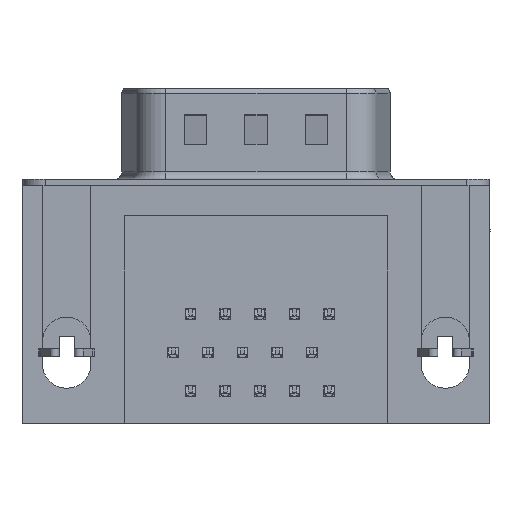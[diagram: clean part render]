
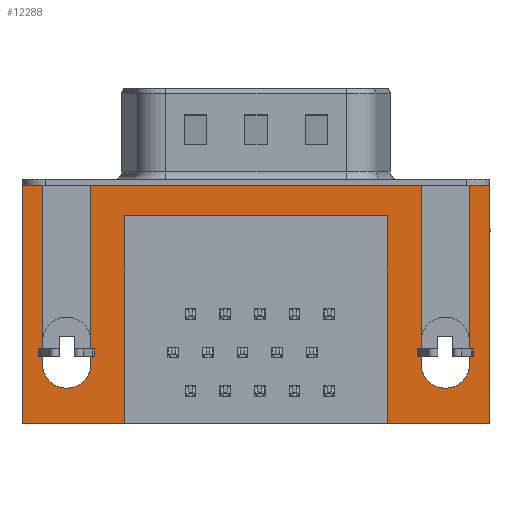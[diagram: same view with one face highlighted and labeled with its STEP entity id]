
A CAD part, front view. The second image highlights one B-rep face of the part: STEP entity #12288.
In plain terms, the highlighted planar face has unit normal (0, -1, 0).
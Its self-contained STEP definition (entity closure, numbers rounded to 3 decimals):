
#37 = DIRECTION ( 'NONE',  ( -1., 0., 0. ) ) ;
#193 = DIRECTION ( 'NONE',  ( 0., 0., 1. ) ) ;
#210 = CARTESIAN_POINT ( 'NONE',  ( 27.9, -6.275, -15.7 ) ) ;
#268 = DIRECTION ( 'NONE',  ( 1., 0., 0. ) ) ;
#341 = CARTESIAN_POINT ( 'NONE',  ( 1.6, -6.275, 0. ) ) ;
#357 = CARTESIAN_POINT ( 'NONE',  ( -2.91, -6.275, -2.5 ) ) ;
#441 = ORIENTED_EDGE ( 'NONE', *, *, #8083, .F. ) ;
#498 = LINE ( 'NONE', #14745, #18078 ) ;
#510 = DIRECTION ( 'NONE',  ( 0., -1., 0. ) ) ;
#714 = VECTOR ( 'NONE', #10806, 1000. ) ;
#1079 = VECTOR ( 'NONE', #17874, 1000. ) ;
#1080 = ORIENTED_EDGE ( 'NONE', *, *, #13354, .F. ) ;
#1344 = CARTESIAN_POINT ( 'NONE',  ( 27.9, -6.275, 0. ) ) ;
#1363 = DIRECTION ( 'NONE',  ( 0., 0., 1. ) ) ;
#1400 = EDGE_CURVE ( 'NONE', #19019, #16526, #22117, .T. ) ;
#1533 = ORIENTED_EDGE ( 'NONE', *, *, #7361, .F. ) ;
#1946 = VECTOR ( 'NONE', #2702, 1000. ) ;
#1990 = ORIENTED_EDGE ( 'NONE', *, *, #1400, .F. ) ;
#2152 = CARTESIAN_POINT ( 'NONE',  ( 1.6, -6.275, 0. ) ) ;
#2352 = DIRECTION ( 'NONE',  ( 1., 0., 0. ) ) ;
#2355 = CARTESIAN_POINT ( 'NONE',  ( -2.91, -6.275, 0. ) ) ;
#2475 = DIRECTION ( 'NONE',  ( 0., 0., 1. ) ) ;
#2587 = DIRECTION ( 'NONE',  ( 0., 0., -1. ) ) ;
#2607 = EDGE_CURVE ( 'NONE', #9757, #21020, #15653, .T. ) ;
#2695 = EDGE_LOOP ( 'NONE', ( #20753, #1080, #9929, #441, #14079, #2718, #10055, #1533, #7491, #19380, #7294, #12088, #5726, #17507, #7734, #5075, #21317, #1990 ) ) ;
#2702 = DIRECTION ( 'NONE',  ( 0., 0., -1. ) ) ;
#2718 = ORIENTED_EDGE ( 'NONE', *, *, #3347, .F. ) ;
#3008 = AXIS2_PLACEMENT_3D ( 'NONE', #4215, #13097, #2587 ) ;
#3164 = CARTESIAN_POINT ( 'NONE',  ( 27.9, -6.275, -15.7 ) ) ;
#3347 = EDGE_CURVE ( 'NONE', #20276, #3388, #16456, .T. ) ;
#3388 = VERTEX_POINT ( 'NONE', #341 ) ;
#3489 = VECTOR ( 'NONE', #19010, 1000. ) ;
#3686 = CARTESIAN_POINT ( 'NONE',  ( 23.39, -6.275, 0. ) ) ;
#3694 = EDGE_CURVE ( 'NONE', #15431, #12203, #18050, .T. ) ;
#3867 = CARTESIAN_POINT ( 'NONE',  ( 24.99, -6.275, -11.78 ) ) ;
#4183 = CARTESIAN_POINT ( 'NONE',  ( -2.91, -6.275, 0. ) ) ;
#4215 = CARTESIAN_POINT ( 'NONE',  ( -2.91, -6.275, -2.5 ) ) ;
#4298 = PLANE ( 'NONE',  #3008 ) ;
#4344 = VECTOR ( 'NONE', #14857, 1000. ) ;
#4402 = CARTESIAN_POINT ( 'NONE',  ( 23.39, -6.275, -11.78 ) ) ;
#4471 = CARTESIAN_POINT ( 'NONE',  ( 26.59, -6.275, -11.78 ) ) ;
#4491 = VERTEX_POINT ( 'NONE', #3686 ) ;
#4549 = EDGE_CURVE ( 'NONE', #3388, #4491, #8476, .T. ) ;
#4665 = CARTESIAN_POINT ( 'NONE',  ( 0., -6.275, -11.78 ) ) ;
#4915 = LINE ( 'NONE', #21211, #714 ) ;
#4988 = EDGE_CURVE ( 'NONE', #21020, #10829, #18798, .T. ) ;
#5075 = ORIENTED_EDGE ( 'NONE', *, *, #2607, .F. ) ;
#5271 = EDGE_CURVE ( 'NONE', #9757, #16526, #8183, .T. ) ;
#5335 = CARTESIAN_POINT ( 'NONE',  ( 3.79, -6.275, -2. ) ) ;
#5635 = DIRECTION ( 'NONE',  ( 0., 0., 1. ) ) ;
#5726 = ORIENTED_EDGE ( 'NONE', *, *, #13194, .F. ) ;
#5757 = VECTOR ( 'NONE', #193, 1000. ) ;
#6047 = VECTOR ( 'NONE', #6522, 1000. ) ;
#6415 = DIRECTION ( 'NONE',  ( 0., 0., -1. ) ) ;
#6522 = DIRECTION ( 'NONE',  ( 0., 0., 1. ) ) ;
#6766 = CARTESIAN_POINT ( 'NONE',  ( 27.9, -6.275, -2.5 ) ) ;
#7183 = LINE ( 'NONE', #18309, #1946 ) ;
#7294 = ORIENTED_EDGE ( 'NONE', *, *, #3694, .F. ) ;
#7361 = EDGE_CURVE ( 'NONE', #18187, #9014, #22047, .T. ) ;
#7491 = ORIENTED_EDGE ( 'NONE', *, *, #17848, .F. ) ;
#7539 = CARTESIAN_POINT ( 'NONE',  ( -2.91, -6.275, -15.7 ) ) ;
#7734 = ORIENTED_EDGE ( 'NONE', *, *, #4988, .F. ) ;
#8083 = EDGE_CURVE ( 'NONE', #4491, #16279, #4915, .T. ) ;
#8183 = LINE ( 'NONE', #6766, #3489 ) ;
#8336 = VERTEX_POINT ( 'NONE', #4471 ) ;
#8476 = LINE ( 'NONE', #4183, #12572 ) ;
#8517 = VECTOR ( 'NONE', #2352, 1000. ) ;
#8565 = CIRCLE ( 'NONE', #20748, 1.6 ) ;
#9014 = VERTEX_POINT ( 'NONE', #17644 ) ;
#9262 = VERTEX_POINT ( 'NONE', #15193 ) ;
#9568 = CARTESIAN_POINT ( 'NONE',  ( 26.59, -6.275, 0. ) ) ;
#9757 = VERTEX_POINT ( 'NONE', #21724 ) ;
#9929 = ORIENTED_EDGE ( 'NONE', *, *, #12757, .F. ) ;
#10055 = ORIENTED_EDGE ( 'NONE', *, *, #15742, .F. ) ;
#10221 = CIRCLE ( 'NONE', #20137, 1.6 ) ;
#10313 = VECTOR ( 'NONE', #13734, 1000. ) ;
#10806 = DIRECTION ( 'NONE',  ( 0., 0., -1. ) ) ;
#10818 = EDGE_CURVE ( 'NONE', #10829, #16124, #11083, .T. ) ;
#10829 = VERTEX_POINT ( 'NONE', #21080 ) ;
#11050 = CARTESIAN_POINT ( 'NONE',  ( 0., -6.275, -11.78 ) ) ;
#11083 = LINE ( 'NONE', #5335, #19821 ) ;
#11266 = CARTESIAN_POINT ( 'NONE',  ( -2.91, -6.275, 0. ) ) ;
#11647 = VERTEX_POINT ( 'NONE', #19538 ) ;
#11906 = DIRECTION ( 'NONE',  ( 0., -1., 0. ) ) ;
#12088 = ORIENTED_EDGE ( 'NONE', *, *, #22444, .F. ) ;
#12150 = DIRECTION ( 'NONE',  ( 1., 0., 0. ) ) ;
#12177 = CARTESIAN_POINT ( 'NONE',  ( 1.6, -6.275, -11.78 ) ) ;
#12203 = VERTEX_POINT ( 'NONE', #2355 ) ;
#12288 = ADVANCED_FACE ( 'NONE', ( #13802 ), #4298, .T. ) ;
#12572 = VECTOR ( 'NONE', #268, 1000. ) ;
#12750 = CARTESIAN_POINT ( 'NONE',  ( 3.79, -6.275, -2. ) ) ;
#12757 = EDGE_CURVE ( 'NONE', #16279, #9262, #10221, .T. ) ;
#12851 = DIRECTION ( 'NONE',  ( 0., 0., -1. ) ) ;
#12874 = CARTESIAN_POINT ( 'NONE',  ( -2.91, -6.275, 0. ) ) ;
#13097 = DIRECTION ( 'NONE',  ( 0., -1., 0. ) ) ;
#13169 = LINE ( 'NONE', #12874, #8517 ) ;
#13194 = EDGE_CURVE ( 'NONE', #16124, #11647, #7183, .T. ) ;
#13354 = EDGE_CURVE ( 'NONE', #9262, #8336, #8565, .T. ) ;
#13376 = AXIS2_PLACEMENT_3D ( 'NONE', #4665, #16907, #6415 ) ;
#13734 = DIRECTION ( 'NONE',  ( -1., 0., 0. ) ) ;
#13802 = FACE_OUTER_BOUND ( 'NONE', #2695, .T. ) ;
#14079 = ORIENTED_EDGE ( 'NONE', *, *, #4549, .F. ) ;
#14366 = EDGE_CURVE ( 'NONE', #12203, #19469, #13169, .T. ) ;
#14745 = CARTESIAN_POINT ( 'NONE',  ( 26.59, -6.275, 0. ) ) ;
#14857 = DIRECTION ( 'NONE',  ( 0., 0., 1. ) ) ;
#15096 = EDGE_CURVE ( 'NONE', #8336, #19019, #498, .T. ) ;
#15098 = CARTESIAN_POINT ( 'NONE',  ( 21.2, -6.275, -15.7 ) ) ;
#15193 = CARTESIAN_POINT ( 'NONE',  ( 24.99, -6.275, -13.38 ) ) ;
#15431 = VERTEX_POINT ( 'NONE', #7539 ) ;
#15653 = LINE ( 'NONE', #210, #1079 ) ;
#15736 = CARTESIAN_POINT ( 'NONE',  ( -1.6, -6.275, 0. ) ) ;
#15742 = EDGE_CURVE ( 'NONE', #9014, #20276, #21002, .T. ) ;
#16114 = DIRECTION ( 'NONE',  ( 0., -1., 0. ) ) ;
#16124 = VERTEX_POINT ( 'NONE', #12750 ) ;
#16279 = VERTEX_POINT ( 'NONE', #4402 ) ;
#16456 = LINE ( 'NONE', #2152, #6047 ) ;
#16526 = VERTEX_POINT ( 'NONE', #1344 ) ;
#16907 = DIRECTION ( 'NONE',  ( 0., -1., 0. ) ) ;
#17486 = DIRECTION ( 'NONE',  ( 0., 0., -1. ) ) ;
#17507 = ORIENTED_EDGE ( 'NONE', *, *, #10818, .F. ) ;
#17539 = CARTESIAN_POINT ( 'NONE',  ( -1.6, -6.275, -11.78 ) ) ;
#17644 = CARTESIAN_POINT ( 'NONE',  ( 0., -6.275, -13.38 ) ) ;
#17848 = EDGE_CURVE ( 'NONE', #19469, #18187, #19594, .T. ) ;
#17872 = VECTOR ( 'NONE', #12150, 1000. ) ;
#17874 = DIRECTION ( 'NONE',  ( -1., 0., 0. ) ) ;
#18050 = LINE ( 'NONE', #357, #5757 ) ;
#18078 = VECTOR ( 'NONE', #2475, 1000. ) ;
#18187 = VERTEX_POINT ( 'NONE', #17539 ) ;
#18309 = CARTESIAN_POINT ( 'NONE',  ( 3.79, -6.275, -2. ) ) ;
#18535 = VECTOR ( 'NONE', #17486, 1000. ) ;
#18798 = LINE ( 'NONE', #19608, #4344 ) ;
#19010 = DIRECTION ( 'NONE',  ( 0., 0., 1. ) ) ;
#19019 = VERTEX_POINT ( 'NONE', #9568 ) ;
#19380 = ORIENTED_EDGE ( 'NONE', *, *, #14366, .F. ) ;
#19469 = VERTEX_POINT ( 'NONE', #20262 ) ;
#19538 = CARTESIAN_POINT ( 'NONE',  ( 3.79, -6.275, -15.7 ) ) ;
#19594 = LINE ( 'NONE', #15736, #18535 ) ;
#19608 = CARTESIAN_POINT ( 'NONE',  ( 21.2, -6.275, -2. ) ) ;
#19821 = VECTOR ( 'NONE', #37, 1000. ) ;
#20137 = AXIS2_PLACEMENT_3D ( 'NONE', #3867, #16114, #5635 ) ;
#20262 = CARTESIAN_POINT ( 'NONE',  ( -1.6, -6.275, 0. ) ) ;
#20276 = VERTEX_POINT ( 'NONE', #12177 ) ;
#20667 = LINE ( 'NONE', #3164, #10313 ) ;
#20748 = AXIS2_PLACEMENT_3D ( 'NONE', #22266, #11906, #1363 ) ;
#20753 = ORIENTED_EDGE ( 'NONE', *, *, #15096, .F. ) ;
#21002 = CIRCLE ( 'NONE', #13376, 1.6 ) ;
#21020 = VERTEX_POINT ( 'NONE', #15098 ) ;
#21080 = CARTESIAN_POINT ( 'NONE',  ( 21.2, -6.275, -2. ) ) ;
#21211 = CARTESIAN_POINT ( 'NONE',  ( 23.39, -6.275, 0. ) ) ;
#21317 = ORIENTED_EDGE ( 'NONE', *, *, #5271, .T. ) ;
#21724 = CARTESIAN_POINT ( 'NONE',  ( 27.9, -6.275, -15.7 ) ) ;
#21747 = AXIS2_PLACEMENT_3D ( 'NONE', #11050, #510, #12851 ) ;
#22047 = CIRCLE ( 'NONE', #21747, 1.6 ) ;
#22117 = LINE ( 'NONE', #11266, #17872 ) ;
#22266 = CARTESIAN_POINT ( 'NONE',  ( 24.99, -6.275, -11.78 ) ) ;
#22444 = EDGE_CURVE ( 'NONE', #11647, #15431, #20667, .T. ) ;
